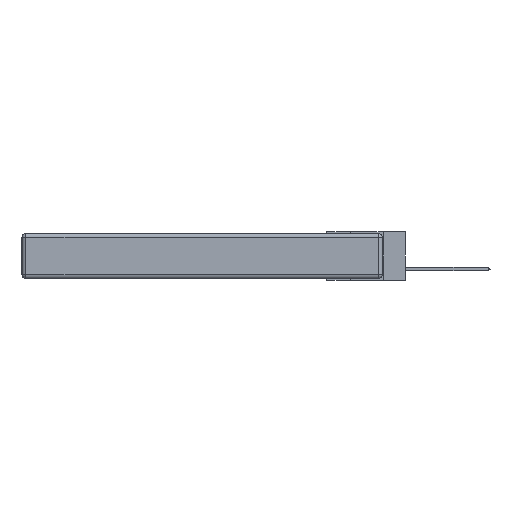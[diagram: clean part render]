
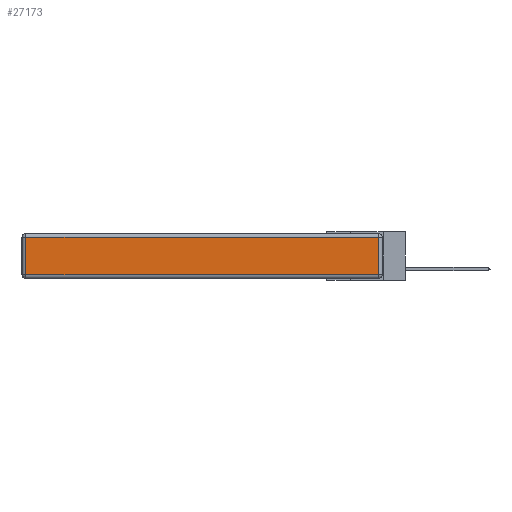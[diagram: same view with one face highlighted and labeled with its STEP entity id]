
A CAD part, left-side view. The second image highlights one B-rep face of the part: STEP entity #27173.
In plain terms, the highlighted planar face has unit normal (-1, 0, 0).
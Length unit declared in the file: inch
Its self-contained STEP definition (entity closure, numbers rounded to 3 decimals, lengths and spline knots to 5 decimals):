
#703 = CARTESIAN_POINT ( 'NONE',  ( 0., 0.03, -0.343 ) ) ;
#998 = DIRECTION ( 'NONE',  ( 0., 0., 1. ) ) ;
#1812 = VECTOR ( 'NONE', #18220, 39.37008 ) ;
#3050 = VERTEX_POINT ( 'NONE', #15794 ) ;
#4149 = CARTESIAN_POINT ( 'NONE',  ( 0., 2.75, -0.03 ) ) ;
#5250 = EDGE_CURVE ( 'NONE', #9091, #20762, #8187, .T. ) ;
#5969 = ORIENTED_EDGE ( 'NONE', *, *, #5250, .T. ) ;
#7578 = ORIENTED_EDGE ( 'NONE', *, *, #17921, .T. ) ;
#7786 = VECTOR ( 'NONE', #998, 39.37008 ) ;
#8187 = LINE ( 'NONE', #29230, #26957 ) ;
#8236 = DIRECTION ( 'NONE',  ( 0., -1., 0. ) ) ;
#8756 = LINE ( 'NONE', #4149, #1812 ) ;
#9081 = VERTEX_POINT ( 'NONE', #22386 ) ;
#9091 = VERTEX_POINT ( 'NONE', #15322 ) ;
#9786 = AXIS2_PLACEMENT_3D ( 'NONE', #28522, #12515, #23893 ) ;
#9877 = CARTESIAN_POINT ( 'NONE',  ( 0., 2.72, -0.343 ) ) ;
#12306 = DIRECTION ( 'NONE',  ( 0., 0., -1. ) ) ;
#12515 = DIRECTION ( 'NONE',  ( -1., 0., 0. ) ) ;
#15322 = CARTESIAN_POINT ( 'NONE',  ( 0., 2.72, -0.313 ) ) ;
#15334 = EDGE_CURVE ( 'NONE', #9081, #9091, #17082, .T. ) ;
#15794 = CARTESIAN_POINT ( 'NONE',  ( 0., 0.03, -0.03 ) ) ;
#15839 = FACE_OUTER_BOUND ( 'NONE', #22177, .T. ) ;
#16796 = PLANE ( 'NONE',  #9786 ) ;
#17082 = LINE ( 'NONE', #9877, #21455 ) ;
#17921 = EDGE_CURVE ( 'NONE', #3050, #9081, #8756, .T. ) ;
#18220 = DIRECTION ( 'NONE',  ( 0., 1., 0. ) ) ;
#18326 = CARTESIAN_POINT ( 'NONE',  ( 0., 0.03, -0.313 ) ) ;
#18827 = LINE ( 'NONE', #703, #7786 ) ;
#19414 = ORIENTED_EDGE ( 'NONE', *, *, #22848, .T. ) ;
#20762 = VERTEX_POINT ( 'NONE', #18326 ) ;
#21455 = VECTOR ( 'NONE', #12306, 39.37008 ) ;
#22177 = EDGE_LOOP ( 'NONE', ( #5969, #19414, #7578, #22384 ) ) ;
#22384 = ORIENTED_EDGE ( 'NONE', *, *, #15334, .T. ) ;
#22386 = CARTESIAN_POINT ( 'NONE',  ( 0., 2.72, -0.03 ) ) ;
#22848 = EDGE_CURVE ( 'NONE', #20762, #3050, #18827, .T. ) ;
#23893 = DIRECTION ( 'NONE',  ( 0., 0., 1. ) ) ;
#26957 = VECTOR ( 'NONE', #8236, 39.37008 ) ;
#27173 = ADVANCED_FACE ( 'NONE', ( #15839 ), #16796, .T. ) ;
#28522 = CARTESIAN_POINT ( 'NONE',  ( 0., 0., -0.343 ) ) ;
#29230 = CARTESIAN_POINT ( 'NONE',  ( 0., 0., -0.313 ) ) ;
